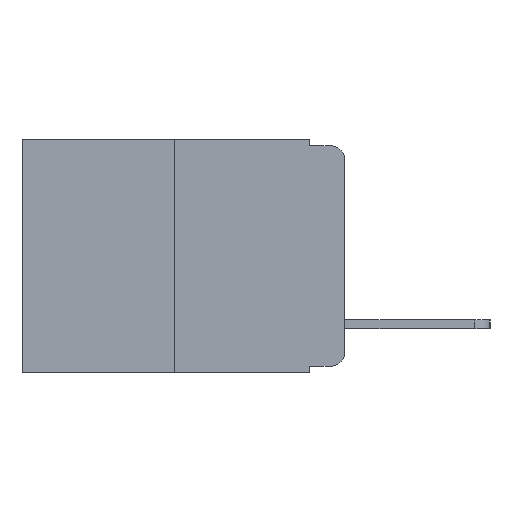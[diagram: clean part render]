
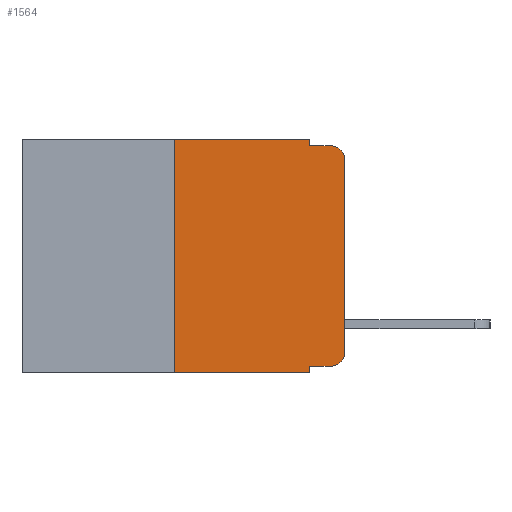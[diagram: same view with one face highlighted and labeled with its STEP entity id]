
A CAD part, left-side view. The second image highlights one B-rep face of the part: STEP entity #1564.
In plain terms, the highlighted planar face has unit normal (-1, 0, 0).
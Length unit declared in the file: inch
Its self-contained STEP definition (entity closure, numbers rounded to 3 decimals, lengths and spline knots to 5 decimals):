
#714 = DIRECTION ( 'NONE',  ( 0., -1., 0. ) ) ;
#881 = VERTEX_POINT ( 'NONE', #19888 ) ;
#1468 = EDGE_CURVE ( 'NONE', #19123, #10722, #21125, .T. ) ;
#1564 = ADVANCED_FACE ( 'NONE', ( #18252 ), #15992, .F. ) ;
#2101 = EDGE_CURVE ( 'NONE', #16046, #2957, #10271, .T. ) ;
#2155 = VECTOR ( 'NONE', #3855, 39.37008 ) ;
#2957 = VERTEX_POINT ( 'NONE', #6550 ) ;
#2983 = CARTESIAN_POINT ( 'NONE',  ( 0., 0., 0. ) ) ;
#3078 = ORIENTED_EDGE ( 'NONE', *, *, #2101, .T. ) ;
#3813 = CARTESIAN_POINT ( 'NONE',  ( 0., 0.02, -0.313 ) ) ;
#3855 = DIRECTION ( 'NONE',  ( 0., -1., 0. ) ) ;
#4199 = CARTESIAN_POINT ( 'NONE',  ( 0., 0.02, -0.333 ) ) ;
#4505 = DIRECTION ( 'NONE',  ( 0., -1., 0. ) ) ;
#4565 = ORIENTED_EDGE ( 'NONE', *, *, #13881, .F. ) ;
#5732 = DIRECTION ( 'NONE',  ( 0., 0., -1. ) ) ;
#5780 = CARTESIAN_POINT ( 'NONE',  ( 0., 0.051, -0.333 ) ) ;
#5968 = DIRECTION ( 'NONE',  ( -1., 0., 0. ) ) ;
#6550 = CARTESIAN_POINT ( 'NONE',  ( 0., 0., -0.313 ) ) ;
#6945 = CARTESIAN_POINT ( 'NONE',  ( 0., 0.473, -0.343 ) ) ;
#7566 = DIRECTION ( 'NONE',  ( 0., 0., -1. ) ) ;
#7721 = VECTOR ( 'NONE', #8723, 39.37008 ) ;
#8084 = CARTESIAN_POINT ( 'NONE',  ( 0., 0.051, 0. ) ) ;
#8723 = DIRECTION ( 'NONE',  ( 0., -1., 0. ) ) ;
#9670 = VECTOR ( 'NONE', #4505, 39.37008 ) ;
#10271 = CIRCLE ( 'NONE', #15371, 0.02 ) ;
#10354 = CARTESIAN_POINT ( 'NONE',  ( 0., 0.051, -0.01 ) ) ;
#10382 = CARTESIAN_POINT ( 'NONE',  ( 0., 0.25, -0.343 ) ) ;
#10431 = EDGE_CURVE ( 'NONE', #2957, #881, #11317, .T. ) ;
#10537 = VERTEX_POINT ( 'NONE', #20675 ) ;
#10722 = VERTEX_POINT ( 'NONE', #18104 ) ;
#10893 = CARTESIAN_POINT ( 'NONE',  ( 0., 0.051, 0. ) ) ;
#10900 = DIRECTION ( 'NONE',  ( 0., 0., -1. ) ) ;
#11101 = ORIENTED_EDGE ( 'NONE', *, *, #14902, .F. ) ;
#11317 = LINE ( 'NONE', #2983, #19682 ) ;
#11643 = ORIENTED_EDGE ( 'NONE', *, *, #15345, .F. ) ;
#11887 = LINE ( 'NONE', #21617, #15360 ) ;
#11917 = LINE ( 'NONE', #5780, #2155 ) ;
#11953 = CARTESIAN_POINT ( 'NONE',  ( 0., 0.02, -0.01 ) ) ;
#12168 = ORIENTED_EDGE ( 'NONE', *, *, #15963, .T. ) ;
#12925 = ORIENTED_EDGE ( 'NONE', *, *, #12987, .T. ) ;
#12975 = VECTOR ( 'NONE', #20755, 39.37008 ) ;
#12987 = EDGE_CURVE ( 'NONE', #881, #16608, #17981, .T. ) ;
#13117 = EDGE_CURVE ( 'NONE', #18357, #16608, #11887, .T. ) ;
#13881 = EDGE_CURVE ( 'NONE', #21754, #18357, #22032, .T. ) ;
#14103 = LINE ( 'NONE', #10893, #12975 ) ;
#14165 = EDGE_CURVE ( 'NONE', #17194, #21754, #22256, .T. ) ;
#14902 = EDGE_CURVE ( 'NONE', #19123, #17194, #21407, .T. ) ;
#15216 = CARTESIAN_POINT ( 'NONE',  ( 0., 0.473, 0. ) ) ;
#15345 = EDGE_CURVE ( 'NONE', #10537, #10722, #14103, .T. ) ;
#15360 = VECTOR ( 'NONE', #714, 39.37008 ) ;
#15371 = AXIS2_PLACEMENT_3D ( 'NONE', #3813, #16285, #5732 ) ;
#15421 = DIRECTION ( 'NONE',  ( 0., 0., 1. ) ) ;
#15504 = AXIS2_PLACEMENT_3D ( 'NONE', #17658, #20758, #10900 ) ;
#15656 = ORIENTED_EDGE ( 'NONE', *, *, #1468, .T. ) ;
#15963 = EDGE_CURVE ( 'NONE', #10537, #16046, #11917, .T. ) ;
#15992 = PLANE ( 'NONE',  #15504 ) ;
#16046 = VERTEX_POINT ( 'NONE', #4199 ) ;
#16285 = DIRECTION ( 'NONE',  ( -1., 0., 0. ) ) ;
#16488 = CARTESIAN_POINT ( 'NONE',  ( 0., 0.02, -0.03 ) ) ;
#16608 = VERTEX_POINT ( 'NONE', #11953 ) ;
#17194 = VERTEX_POINT ( 'NONE', #19717 ) ;
#17275 = VECTOR ( 'NONE', #22135, 39.37008 ) ;
#17658 = CARTESIAN_POINT ( 'NONE',  ( 0., 0.473, 0. ) ) ;
#17922 = CARTESIAN_POINT ( 'NONE',  ( 0., 0.051, 0. ) ) ;
#17981 = CIRCLE ( 'NONE', #21159, 0.02 ) ;
#18104 = CARTESIAN_POINT ( 'NONE',  ( 0., 0.051, -0.343 ) ) ;
#18119 = DIRECTION ( 'NONE',  ( 0., 0., -1. ) ) ;
#18252 = FACE_OUTER_BOUND ( 'NONE', #20590, .T. ) ;
#18357 = VERTEX_POINT ( 'NONE', #10354 ) ;
#18453 = VECTOR ( 'NONE', #7566, 39.37008 ) ;
#18985 = ORIENTED_EDGE ( 'NONE', *, *, #14165, .F. ) ;
#19123 = VERTEX_POINT ( 'NONE', #10382 ) ;
#19682 = VECTOR ( 'NONE', #15421, 39.37008 ) ;
#19717 = CARTESIAN_POINT ( 'NONE',  ( 0., 0.25, 0. ) ) ;
#19888 = CARTESIAN_POINT ( 'NONE',  ( 0., 0., -0.03 ) ) ;
#20590 = EDGE_LOOP ( 'NONE', ( #21119, #12925, #21619, #4565, #18985, #11101, #15656, #11643, #12168, #3078 ) ) ;
#20598 = CARTESIAN_POINT ( 'NONE',  ( 0., 0.25, 0. ) ) ;
#20675 = CARTESIAN_POINT ( 'NONE',  ( 0., 0.051, -0.333 ) ) ;
#20755 = DIRECTION ( 'NONE',  ( 0., 0., -1. ) ) ;
#20758 = DIRECTION ( 'NONE',  ( 1., 0., 0. ) ) ;
#21119 = ORIENTED_EDGE ( 'NONE', *, *, #10431, .T. ) ;
#21125 = LINE ( 'NONE', #6945, #7721 ) ;
#21159 = AXIS2_PLACEMENT_3D ( 'NONE', #16488, #5968, #18119 ) ;
#21407 = LINE ( 'NONE', #20598, #17275 ) ;
#21617 = CARTESIAN_POINT ( 'NONE',  ( 0., 0.051, -0.01 ) ) ;
#21619 = ORIENTED_EDGE ( 'NONE', *, *, #13117, .F. ) ;
#21754 = VERTEX_POINT ( 'NONE', #8084 ) ;
#22032 = LINE ( 'NONE', #17922, #18453 ) ;
#22135 = DIRECTION ( 'NONE',  ( 0., 0., 1. ) ) ;
#22256 = LINE ( 'NONE', #15216, #9670 ) ;
